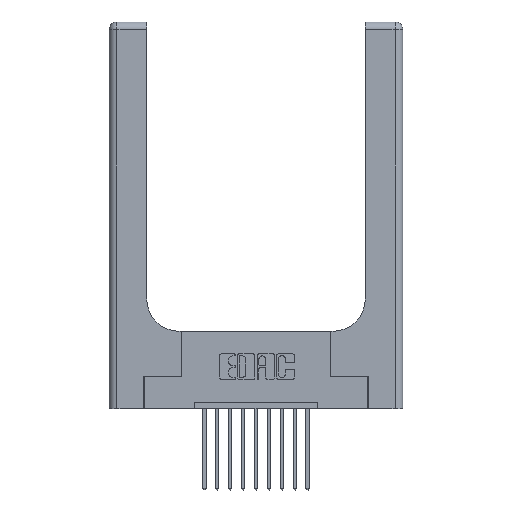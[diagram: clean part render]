
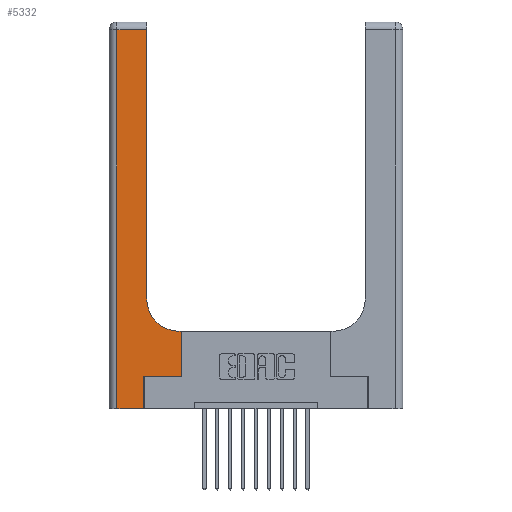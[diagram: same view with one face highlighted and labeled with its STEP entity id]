
A CAD part, top view. The second image highlights one B-rep face of the part: STEP entity #5332.
In plain terms, the highlighted planar face has unit normal (0, 0, 1).
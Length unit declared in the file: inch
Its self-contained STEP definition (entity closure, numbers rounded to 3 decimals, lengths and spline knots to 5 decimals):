
#41 = LINE ( 'NONE', #3805, #4000 ) ;
#43 = LINE ( 'NONE', #12165, #12771 ) ;
#212 = VECTOR ( 'NONE', #14704, 39.37008 ) ;
#435 = VECTOR ( 'NONE', #2184, 39.37008 ) ;
#976 = EDGE_CURVE ( 'NONE', #16284, #16049, #11171, .T. ) ;
#1014 = CARTESIAN_POINT ( 'NONE',  ( 0.2915, 0.6, 0.37 ) ) ;
#1030 = LINE ( 'NONE', #1014, #8211 ) ;
#1569 = ORIENTED_EDGE ( 'NONE', *, *, #3291, .T. ) ;
#1595 = EDGE_LOOP ( 'NONE', ( #3678, #4389, #10968, #7292, #9151, #1569, #14587, #7508, #8692 ) ) ;
#1712 = DIRECTION ( 'NONE',  ( 0., 1., 0. ) ) ;
#2002 = LINE ( 'NONE', #9774, #435 ) ;
#2184 = DIRECTION ( 'NONE',  ( 1., 0., 0. ) ) ;
#2283 = AXIS2_PLACEMENT_3D ( 'NONE', #2459, #2523, #10110 ) ;
#2459 = CARTESIAN_POINT ( 'NONE',  ( 0.5415, 0.85, 0.37 ) ) ;
#2523 = DIRECTION ( 'NONE',  ( 0., 0., -1. ) ) ;
#3022 = CARTESIAN_POINT ( 'NONE',  ( 0.06, 0., 0.37 ) ) ;
#3042 = CIRCLE ( 'NONE', #2283, 0.25 ) ;
#3192 = CARTESIAN_POINT ( 'NONE',  ( 0.2915, 0.85, 0.37 ) ) ;
#3291 = EDGE_CURVE ( 'NONE', #16049, #8297, #2002, .T. ) ;
#3615 = VERTEX_POINT ( 'NONE', #3192 ) ;
#3678 = ORIENTED_EDGE ( 'NONE', *, *, #8831, .T. ) ;
#3698 = EDGE_CURVE ( 'NONE', #8309, #14998, #10896, .T. ) ;
#3805 = CARTESIAN_POINT ( 'NONE',  ( 0.2915, 3., 0.37 ) ) ;
#3812 = CARTESIAN_POINT ( 'NONE',  ( 0., 3., 0.37 ) ) ;
#4000 = VECTOR ( 'NONE', #1712, 39.37008 ) ;
#4371 = VERTEX_POINT ( 'NONE', #13754 ) ;
#4389 = ORIENTED_EDGE ( 'NONE', *, *, #15481, .T. ) ;
#4437 = VECTOR ( 'NONE', #6374, 39.37008 ) ;
#5063 = CARTESIAN_POINT ( 'NONE',  ( 0.5585, 0.25, 0.37 ) ) ;
#5332 = ADVANCED_FACE ( 'NONE', ( #8705 ), #12531, .F. ) ;
#5611 = VECTOR ( 'NONE', #11710, 39.37008 ) ;
#5754 = VERTEX_POINT ( 'NONE', #12951 ) ;
#5873 = EDGE_CURVE ( 'NONE', #8297, #4371, #14397, .T. ) ;
#6069 = VECTOR ( 'NONE', #8781, 39.37008 ) ;
#6374 = DIRECTION ( 'NONE',  ( 0., 1., 0. ) ) ;
#7150 = CARTESIAN_POINT ( 'NONE',  ( 0.5585, 0.25, 0.37 ) ) ;
#7212 = LINE ( 'NONE', #13850, #5611 ) ;
#7292 = ORIENTED_EDGE ( 'NONE', *, *, #14472, .T. ) ;
#7303 = DIRECTION ( 'NONE',  ( -1., 0., 0. ) ) ;
#7508 = ORIENTED_EDGE ( 'NONE', *, *, #14691, .T. ) ;
#8211 = VECTOR ( 'NONE', #7303, 39.37008 ) ;
#8297 = VERTEX_POINT ( 'NONE', #7150 ) ;
#8309 = VERTEX_POINT ( 'NONE', #10665 ) ;
#8369 = DIRECTION ( 'NONE',  ( 1., 0., 0. ) ) ;
#8692 = ORIENTED_EDGE ( 'NONE', *, *, #8946, .T. ) ;
#8705 = FACE_OUTER_BOUND ( 'NONE', #1595, .T. ) ;
#8781 = DIRECTION ( 'NONE',  ( 0., 1., 0. ) ) ;
#8831 = EDGE_CURVE ( 'NONE', #3615, #15011, #41, .T. ) ;
#8946 = EDGE_CURVE ( 'NONE', #5754, #3615, #3042, .T. ) ;
#9151 = ORIENTED_EDGE ( 'NONE', *, *, #976, .T. ) ;
#9279 = CARTESIAN_POINT ( 'NONE',  ( 0.2915, 2.94, 0.37 ) ) ;
#9774 = CARTESIAN_POINT ( 'NONE',  ( 0.269, 0.25, 0.37 ) ) ;
#10110 = DIRECTION ( 'NONE',  ( 1., 0., 0. ) ) ;
#10665 = CARTESIAN_POINT ( 'NONE',  ( 0.06, 2.94, 0.37 ) ) ;
#10879 = CARTESIAN_POINT ( 'NONE',  ( 0.06, 3., 0.37 ) ) ;
#10896 = LINE ( 'NONE', #10879, #212 ) ;
#10968 = ORIENTED_EDGE ( 'NONE', *, *, #3698, .T. ) ;
#11171 = LINE ( 'NONE', #11584, #4437 ) ;
#11584 = CARTESIAN_POINT ( 'NONE',  ( 0.269, 0., 0.37 ) ) ;
#11710 = DIRECTION ( 'NONE',  ( -1., 0., 0. ) ) ;
#12165 = CARTESIAN_POINT ( 'NONE',  ( 0., 0., 0.37 ) ) ;
#12531 = PLANE ( 'NONE',  #13934 ) ;
#12771 = VECTOR ( 'NONE', #8369, 39.37008 ) ;
#12926 = CARTESIAN_POINT ( 'NONE',  ( 0.269, 0.25, 0.37 ) ) ;
#12951 = CARTESIAN_POINT ( 'NONE',  ( 0.5415, 0.6, 0.37 ) ) ;
#13466 = CARTESIAN_POINT ( 'NONE',  ( 0.269, 0., 0.37 ) ) ;
#13754 = CARTESIAN_POINT ( 'NONE',  ( 0.5585, 0.6, 0.37 ) ) ;
#13850 = CARTESIAN_POINT ( 'NONE',  ( 0., 2.94, 0.37 ) ) ;
#13934 = AXIS2_PLACEMENT_3D ( 'NONE', #3812, #16289, #16391 ) ;
#14397 = LINE ( 'NONE', #5063, #6069 ) ;
#14472 = EDGE_CURVE ( 'NONE', #14998, #16284, #43, .T. ) ;
#14587 = ORIENTED_EDGE ( 'NONE', *, *, #5873, .T. ) ;
#14691 = EDGE_CURVE ( 'NONE', #4371, #5754, #1030, .T. ) ;
#14704 = DIRECTION ( 'NONE',  ( 0., -1., 0. ) ) ;
#14998 = VERTEX_POINT ( 'NONE', #3022 ) ;
#15011 = VERTEX_POINT ( 'NONE', #9279 ) ;
#15481 = EDGE_CURVE ( 'NONE', #15011, #8309, #7212, .T. ) ;
#16049 = VERTEX_POINT ( 'NONE', #12926 ) ;
#16284 = VERTEX_POINT ( 'NONE', #13466 ) ;
#16289 = DIRECTION ( 'NONE',  ( 0., 0., -1. ) ) ;
#16391 = DIRECTION ( 'NONE',  ( -1., 0., 0. ) ) ;
